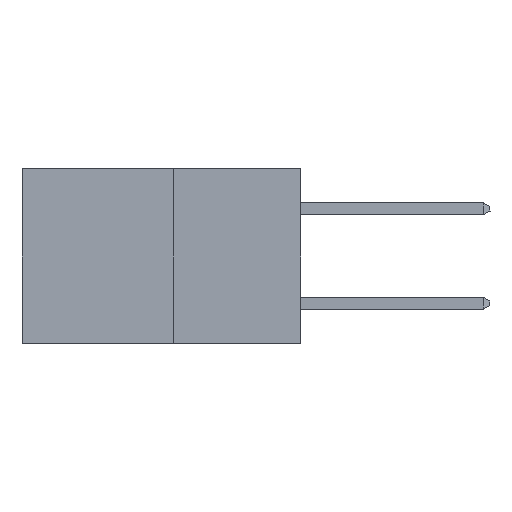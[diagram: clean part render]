
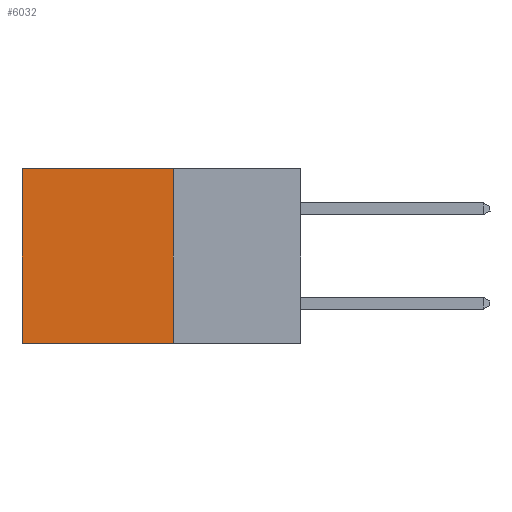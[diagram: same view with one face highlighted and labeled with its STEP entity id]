
A CAD part, left-side view. The second image highlights one B-rep face of the part: STEP entity #6032.
In plain terms, the highlighted planar face has unit normal (-1, 0, 0).
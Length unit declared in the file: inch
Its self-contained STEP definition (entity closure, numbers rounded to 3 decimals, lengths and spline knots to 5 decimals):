
#3322 = ORIENTED_EDGE ( 'NONE', *, *, #21820, .F. ) ;
#4415 = CARTESIAN_POINT ( 'NONE',  ( 0.277, 0.27, -0.37 ) ) ;
#4777 = VECTOR ( 'NONE', #11190, 39.37008 ) ;
#6032 = ADVANCED_FACE ( 'NONE', ( #8279 ), #30202, .F. ) ;
#6928 = VERTEX_POINT ( 'NONE', #4415 ) ;
#7105 = VECTOR ( 'NONE', #13306, 39.37008 ) ;
#7977 = LINE ( 'NONE', #35079, #7105 ) ;
#8279 = FACE_OUTER_BOUND ( 'NONE', #20391, .T. ) ;
#8509 = CARTESIAN_POINT ( 'NONE',  ( 0.277, 0.27, -0.37 ) ) ;
#9845 = VECTOR ( 'NONE', #30158, 39.37008 ) ;
#10582 = CARTESIAN_POINT ( 'NONE',  ( 0.277, 0.27, -0.37 ) ) ;
#11190 = DIRECTION ( 'NONE',  ( 0., 0., -1. ) ) ;
#13306 = DIRECTION ( 'NONE',  ( 0., 1., 0. ) ) ;
#15574 = VERTEX_POINT ( 'NONE', #22122 ) ;
#17178 = LINE ( 'NONE', #10582, #23708 ) ;
#17850 = CARTESIAN_POINT ( 'NONE',  ( 0.277, 0.59, 0. ) ) ;
#18623 = EDGE_CURVE ( 'NONE', #26257, #30826, #31497, .T. ) ;
#20391 = EDGE_LOOP ( 'NONE', ( #34281, #3322, #24514, #26862 ) ) ;
#20979 = AXIS2_PLACEMENT_3D ( 'NONE', #30008, #29975, #29828 ) ;
#21467 = DIRECTION ( 'NONE',  ( 0., 1., 0. ) ) ;
#21820 = EDGE_CURVE ( 'NONE', #6928, #30826, #17178, .T. ) ;
#22122 = CARTESIAN_POINT ( 'NONE',  ( 0.277, 0.27, 0. ) ) ;
#22432 = CARTESIAN_POINT ( 'NONE',  ( 0.277, 0.59, -0.37 ) ) ;
#23708 = VECTOR ( 'NONE', #21467, 39.37008 ) ;
#23843 = EDGE_CURVE ( 'NONE', #15574, #6928, #26551, .T. ) ;
#24514 = ORIENTED_EDGE ( 'NONE', *, *, #23843, .F. ) ;
#26257 = VERTEX_POINT ( 'NONE', #17850 ) ;
#26551 = LINE ( 'NONE', #8509, #4777 ) ;
#26862 = ORIENTED_EDGE ( 'NONE', *, *, #28016, .T. ) ;
#27461 = CARTESIAN_POINT ( 'NONE',  ( 0.277, 0.59, -0.37 ) ) ;
#28016 = EDGE_CURVE ( 'NONE', #15574, #26257, #7977, .T. ) ;
#29828 = DIRECTION ( 'NONE',  ( 0., 0., -1. ) ) ;
#29975 = DIRECTION ( 'NONE',  ( 1., 0., 0. ) ) ;
#30008 = CARTESIAN_POINT ( 'NONE',  ( 0.277, 0.27, -0.37 ) ) ;
#30158 = DIRECTION ( 'NONE',  ( 0., 0., -1. ) ) ;
#30202 = PLANE ( 'NONE',  #20979 ) ;
#30826 = VERTEX_POINT ( 'NONE', #22432 ) ;
#31497 = LINE ( 'NONE', #27461, #9845 ) ;
#34281 = ORIENTED_EDGE ( 'NONE', *, *, #18623, .T. ) ;
#35079 = CARTESIAN_POINT ( 'NONE',  ( 0.277, 0.27, 0. ) ) ;
